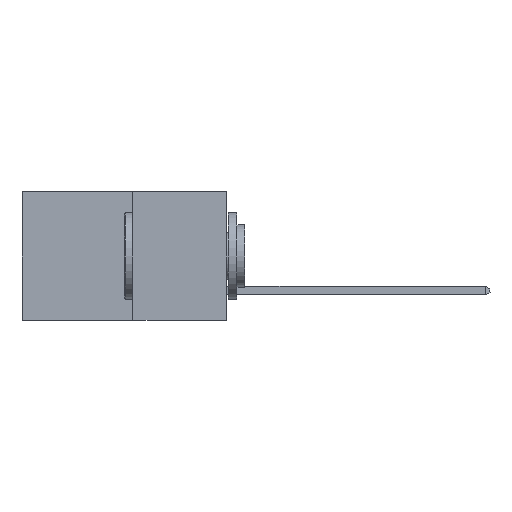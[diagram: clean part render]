
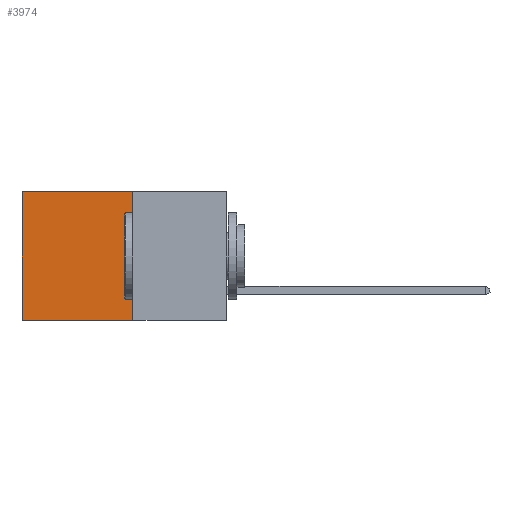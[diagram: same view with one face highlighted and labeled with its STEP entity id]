
A CAD part, left-side view. The second image highlights one B-rep face of the part: STEP entity #3974.
In plain terms, the highlighted planar face has unit normal (-1, 0, 0).
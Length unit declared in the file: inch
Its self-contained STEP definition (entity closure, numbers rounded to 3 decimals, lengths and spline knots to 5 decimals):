
#84 = CARTESIAN_POINT ( 'NONE',  ( 0.277, 0.59, -0.37 ) ) ;
#290 = VERTEX_POINT ( 'NONE', #5522 ) ;
#329 = CARTESIAN_POINT ( 'NONE',  ( 0.277, 0.27, 0. ) ) ;
#1053 = VECTOR ( 'NONE', #11403, 39.37008 ) ;
#2454 = DIRECTION ( 'NONE',  ( 0., 0., -1. ) ) ;
#2555 = CARTESIAN_POINT ( 'NONE',  ( 0.277, 0.27, -0.37 ) ) ;
#3047 = ORIENTED_EDGE ( 'NONE', *, *, #5832, .T. ) ;
#3108 = CARTESIAN_POINT ( 'NONE',  ( 0.277, 0.59, 0. ) ) ;
#3722 = LINE ( 'NONE', #11556, #10697 ) ;
#3974 = ADVANCED_FACE ( 'NONE', ( #8080 ), #6239, .F. ) ;
#4275 = VERTEX_POINT ( 'NONE', #3108 ) ;
#4989 = CARTESIAN_POINT ( 'NONE',  ( 0.277, 0.59, -0.37 ) ) ;
#5401 = ORIENTED_EDGE ( 'NONE', *, *, #8276, .F. ) ;
#5522 = CARTESIAN_POINT ( 'NONE',  ( 0.277, 0.27, -0.37 ) ) ;
#5693 = AXIS2_PLACEMENT_3D ( 'NONE', #6281, #6191, #6189 ) ;
#5832 = EDGE_CURVE ( 'NONE', #9500, #4275, #11891, .T. ) ;
#6189 = DIRECTION ( 'NONE',  ( 0., 0., -1. ) ) ;
#6191 = DIRECTION ( 'NONE',  ( 1., 0., 0. ) ) ;
#6239 = PLANE ( 'NONE',  #5693 ) ;
#6281 = CARTESIAN_POINT ( 'NONE',  ( 0.277, 0.27, -0.37 ) ) ;
#7357 = ORIENTED_EDGE ( 'NONE', *, *, #8466, .T. ) ;
#7994 = DIRECTION ( 'NONE',  ( 0., 0., -1. ) ) ;
#8080 = FACE_OUTER_BOUND ( 'NONE', #10625, .T. ) ;
#8276 = EDGE_CURVE ( 'NONE', #9500, #290, #11208, .T. ) ;
#8466 = EDGE_CURVE ( 'NONE', #4275, #9193, #11912, .T. ) ;
#8775 = VECTOR ( 'NONE', #2454, 39.37008 ) ;
#9193 = VERTEX_POINT ( 'NONE', #4989 ) ;
#9471 = VECTOR ( 'NONE', #7994, 39.37008 ) ;
#9500 = VERTEX_POINT ( 'NONE', #329 ) ;
#9781 = ORIENTED_EDGE ( 'NONE', *, *, #10124, .F. ) ;
#10124 = EDGE_CURVE ( 'NONE', #290, #9193, #3722, .T. ) ;
#10625 = EDGE_LOOP ( 'NONE', ( #7357, #9781, #5401, #3047 ) ) ;
#10697 = VECTOR ( 'NONE', #11607, 39.37008 ) ;
#11208 = LINE ( 'NONE', #2555, #8775 ) ;
#11403 = DIRECTION ( 'NONE',  ( 0., 1., 0. ) ) ;
#11556 = CARTESIAN_POINT ( 'NONE',  ( 0.277, 0.27, -0.37 ) ) ;
#11571 = CARTESIAN_POINT ( 'NONE',  ( 0.277, 0.27, 0. ) ) ;
#11607 = DIRECTION ( 'NONE',  ( 0., 1., 0. ) ) ;
#11891 = LINE ( 'NONE', #11571, #1053 ) ;
#11912 = LINE ( 'NONE', #84, #9471 ) ;
